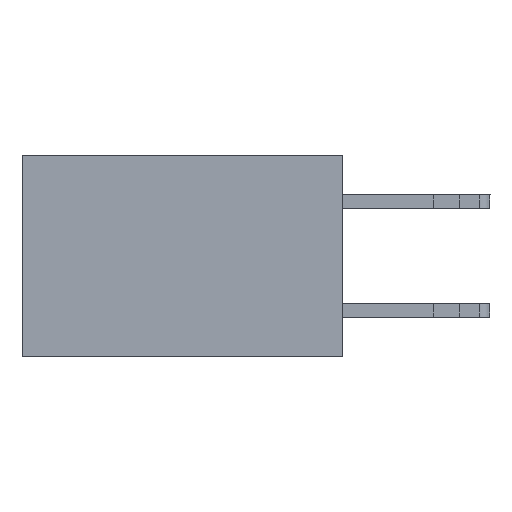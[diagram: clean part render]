
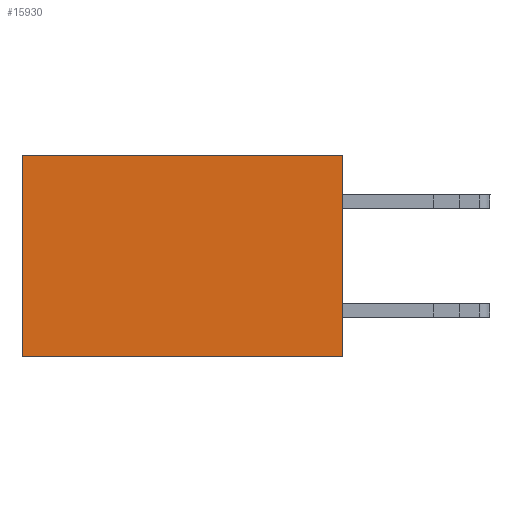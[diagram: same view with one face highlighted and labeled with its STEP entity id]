
A CAD part, left-side view. The second image highlights one B-rep face of the part: STEP entity #15930.
In plain terms, the highlighted planar face has unit normal (-1, 0, 0).
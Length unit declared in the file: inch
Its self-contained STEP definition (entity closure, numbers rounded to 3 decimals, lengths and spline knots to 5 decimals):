
#17 = DIRECTION ( 'NONE',  ( 0., 1., 0. ) ) ;
#604 = VECTOR ( 'NONE', #17, 39.37008 ) ;
#820 = DIRECTION ( 'NONE',  ( 0., 0., -1. ) ) ;
#831 = ORIENTED_EDGE ( 'NONE', *, *, #10875, .F. ) ;
#868 = CARTESIAN_POINT ( 'NONE',  ( 0.277, 0.59, 0. ) ) ;
#1204 = DIRECTION ( 'NONE',  ( 1., 0., 0. ) ) ;
#1455 = EDGE_CURVE ( 'NONE', #3859, #17903, #12215, .T. ) ;
#3094 = CARTESIAN_POINT ( 'NONE',  ( 0.277, 0.59, -0.37 ) ) ;
#3102 = CARTESIAN_POINT ( 'NONE',  ( 0.277, 0., -0.37 ) ) ;
#3191 = AXIS2_PLACEMENT_3D ( 'NONE', #13715, #1204, #12460 ) ;
#3417 = ORIENTED_EDGE ( 'NONE', *, *, #17629, .F. ) ;
#3859 = VERTEX_POINT ( 'NONE', #868 ) ;
#4361 = DIRECTION ( 'NONE',  ( 0., 0., -1. ) ) ;
#5568 = DIRECTION ( 'NONE',  ( 0., 1., 0. ) ) ;
#7912 = VERTEX_POINT ( 'NONE', #20074 ) ;
#8715 = VERTEX_POINT ( 'NONE', #11760 ) ;
#8886 = CARTESIAN_POINT ( 'NONE',  ( 0.277, 0., 0. ) ) ;
#8939 = VECTOR ( 'NONE', #5568, 39.37008 ) ;
#8961 = EDGE_LOOP ( 'NONE', ( #9442, #831, #3417, #11883 ) ) ;
#9164 = PLANE ( 'NONE',  #3191 ) ;
#9442 = ORIENTED_EDGE ( 'NONE', *, *, #1455, .T. ) ;
#10317 = LINE ( 'NONE', #8886, #8939 ) ;
#10875 = EDGE_CURVE ( 'NONE', #8715, #17903, #14864, .T. ) ;
#11760 = CARTESIAN_POINT ( 'NONE',  ( 0.277, 0., -0.37 ) ) ;
#11883 = ORIENTED_EDGE ( 'NONE', *, *, #17509, .T. ) ;
#12215 = LINE ( 'NONE', #18525, #15878 ) ;
#12460 = DIRECTION ( 'NONE',  ( 0., 0., -1. ) ) ;
#13715 = CARTESIAN_POINT ( 'NONE',  ( 0.277, 0., -0.37 ) ) ;
#14864 = LINE ( 'NONE', #3102, #604 ) ;
#14981 = CARTESIAN_POINT ( 'NONE',  ( 0.277, 0., -0.37 ) ) ;
#15878 = VECTOR ( 'NONE', #4361, 39.37008 ) ;
#15930 = ADVANCED_FACE ( 'NONE', ( #16915 ), #9164, .F. ) ;
#16434 = LINE ( 'NONE', #14981, #16868 ) ;
#16868 = VECTOR ( 'NONE', #820, 39.37008 ) ;
#16915 = FACE_OUTER_BOUND ( 'NONE', #8961, .T. ) ;
#17509 = EDGE_CURVE ( 'NONE', #7912, #3859, #10317, .T. ) ;
#17629 = EDGE_CURVE ( 'NONE', #7912, #8715, #16434, .T. ) ;
#17903 = VERTEX_POINT ( 'NONE', #3094 ) ;
#18525 = CARTESIAN_POINT ( 'NONE',  ( 0.277, 0.59, -0.37 ) ) ;
#20074 = CARTESIAN_POINT ( 'NONE',  ( 0.277, 0., 0. ) ) ;
